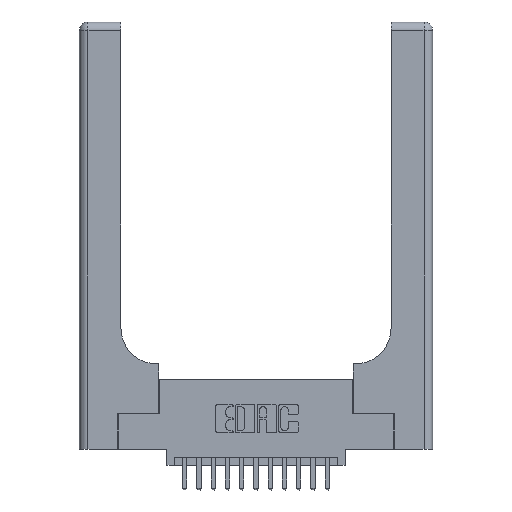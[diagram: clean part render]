
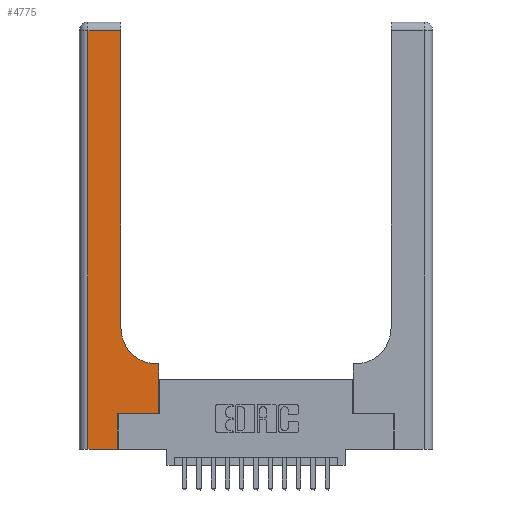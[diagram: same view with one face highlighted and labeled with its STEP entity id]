
A CAD part, top view. The second image highlights one B-rep face of the part: STEP entity #4775.
In plain terms, the highlighted planar face has unit normal (0, 0, 1).
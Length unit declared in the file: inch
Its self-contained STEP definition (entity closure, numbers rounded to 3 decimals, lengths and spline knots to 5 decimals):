
#497 = EDGE_CURVE ( 'NONE', #1761, #15109, #11783, .T. ) ;
#659 = DIRECTION ( 'NONE',  ( -1., 0., 0. ) ) ;
#733 = LINE ( 'NONE', #9240, #1203 ) ;
#1203 = VECTOR ( 'NONE', #659, 39.37008 ) ;
#1318 = DIRECTION ( 'NONE',  ( 0., 1., 0. ) ) ;
#1379 = CARTESIAN_POINT ( 'NONE',  ( 0., 2.94, 0.37 ) ) ;
#1761 = VERTEX_POINT ( 'NONE', #6984 ) ;
#1827 = LINE ( 'NONE', #14143, #13126 ) ;
#2099 = VERTEX_POINT ( 'NONE', #3879 ) ;
#2332 = DIRECTION ( 'NONE',  ( 0., 1., 0. ) ) ;
#2376 = VECTOR ( 'NONE', #1318, 39.37008 ) ;
#2440 = LINE ( 'NONE', #10809, #13709 ) ;
#2558 = VECTOR ( 'NONE', #11317, 39.37008 ) ;
#2577 = CIRCLE ( 'NONE', #3922, 0.25 ) ;
#2623 = PLANE ( 'NONE',  #12134 ) ;
#3007 = LINE ( 'NONE', #1379, #2558 ) ;
#3859 = VECTOR ( 'NONE', #8879, 39.37008 ) ;
#3879 = CARTESIAN_POINT ( 'NONE',  ( 0.5585, 0.6, 0.37 ) ) ;
#3919 = DIRECTION ( 'NONE',  ( 1., 0., 0. ) ) ;
#3922 = AXIS2_PLACEMENT_3D ( 'NONE', #13726, #5308, #15121 ) ;
#3931 = CARTESIAN_POINT ( 'NONE',  ( 0., 0., 0.37 ) ) ;
#3990 = DIRECTION ( 'NONE',  ( 1., 0., 0. ) ) ;
#4253 = DIRECTION ( 'NONE',  ( 0., -1., 0. ) ) ;
#4258 = CARTESIAN_POINT ( 'NONE',  ( 0.5585, 0.25, 0.37 ) ) ;
#4658 = VERTEX_POINT ( 'NONE', #6550 ) ;
#4775 = ADVANCED_FACE ( 'NONE', ( #17881 ), #2623, .F. ) ;
#5308 = DIRECTION ( 'NONE',  ( 0., 0., -1. ) ) ;
#5500 = CARTESIAN_POINT ( 'NONE',  ( 0.269, 0.25, 0.37 ) ) ;
#5503 = DIRECTION ( 'NONE',  ( 0., 0., -1. ) ) ;
#6205 = VECTOR ( 'NONE', #3990, 39.37008 ) ;
#6450 = CARTESIAN_POINT ( 'NONE',  ( 0.2915, 2.94, 0.37 ) ) ;
#6550 = CARTESIAN_POINT ( 'NONE',  ( 0.5585, 0.25, 0.37 ) ) ;
#6673 = EDGE_CURVE ( 'NONE', #6721, #1761, #17290, .T. ) ;
#6721 = VERTEX_POINT ( 'NONE', #6948 ) ;
#6804 = EDGE_LOOP ( 'NONE', ( #8723, #9300, #10432, #13533, #15608, #15686, #16881, #18004, #18183 ) ) ;
#6948 = CARTESIAN_POINT ( 'NONE',  ( 0.06, 0., 0.37 ) ) ;
#6984 = CARTESIAN_POINT ( 'NONE',  ( 0.269, 0., 0.37 ) ) ;
#7902 = EDGE_CURVE ( 'NONE', #16306, #13598, #2577, .T. ) ;
#8066 = CARTESIAN_POINT ( 'NONE',  ( 0.269, 0.25, 0.37 ) ) ;
#8712 = CARTESIAN_POINT ( 'NONE',  ( 0.269, 0., 0.37 ) ) ;
#8723 = ORIENTED_EDGE ( 'NONE', *, *, #12403, .T. ) ;
#8879 = DIRECTION ( 'NONE',  ( 0., 1., 0. ) ) ;
#9089 = EDGE_CURVE ( 'NONE', #12376, #11332, #3007, .T. ) ;
#9240 = CARTESIAN_POINT ( 'NONE',  ( 0.2915, 0.6, 0.37 ) ) ;
#9300 = ORIENTED_EDGE ( 'NONE', *, *, #9089, .T. ) ;
#9373 = CARTESIAN_POINT ( 'NONE',  ( 0.06, 2.94, 0.37 ) ) ;
#9928 = VECTOR ( 'NONE', #3919, 39.37008 ) ;
#10432 = ORIENTED_EDGE ( 'NONE', *, *, #16872, .T. ) ;
#10809 = CARTESIAN_POINT ( 'NONE',  ( 0.2915, 3., 0.37 ) ) ;
#11226 = CARTESIAN_POINT ( 'NONE',  ( 0.5415, 0.6, 0.37 ) ) ;
#11317 = DIRECTION ( 'NONE',  ( -1., 0., 0. ) ) ;
#11332 = VERTEX_POINT ( 'NONE', #9373 ) ;
#11783 = LINE ( 'NONE', #8712, #3859 ) ;
#12134 = AXIS2_PLACEMENT_3D ( 'NONE', #13912, #5503, #15293 ) ;
#12376 = VERTEX_POINT ( 'NONE', #6450 ) ;
#12403 = EDGE_CURVE ( 'NONE', #13598, #12376, #2440, .T. ) ;
#13126 = VECTOR ( 'NONE', #4253, 39.37008 ) ;
#13533 = ORIENTED_EDGE ( 'NONE', *, *, #6673, .T. ) ;
#13598 = VERTEX_POINT ( 'NONE', #16106 ) ;
#13709 = VECTOR ( 'NONE', #2332, 39.37008 ) ;
#13726 = CARTESIAN_POINT ( 'NONE',  ( 0.5415, 0.85, 0.37 ) ) ;
#13851 = EDGE_CURVE ( 'NONE', #15109, #4658, #17283, .T. ) ;
#13912 = CARTESIAN_POINT ( 'NONE',  ( 0., 3., 0.37 ) ) ;
#14143 = CARTESIAN_POINT ( 'NONE',  ( 0.06, 3., 0.37 ) ) ;
#15109 = VERTEX_POINT ( 'NONE', #5500 ) ;
#15121 = DIRECTION ( 'NONE',  ( 1., 0., 0. ) ) ;
#15155 = EDGE_CURVE ( 'NONE', #4658, #2099, #16009, .T. ) ;
#15293 = DIRECTION ( 'NONE',  ( -1., 0., 0. ) ) ;
#15414 = EDGE_CURVE ( 'NONE', #2099, #16306, #733, .T. ) ;
#15608 = ORIENTED_EDGE ( 'NONE', *, *, #497, .T. ) ;
#15686 = ORIENTED_EDGE ( 'NONE', *, *, #13851, .T. ) ;
#16009 = LINE ( 'NONE', #4258, #2376 ) ;
#16106 = CARTESIAN_POINT ( 'NONE',  ( 0.2915, 0.85, 0.37 ) ) ;
#16306 = VERTEX_POINT ( 'NONE', #11226 ) ;
#16872 = EDGE_CURVE ( 'NONE', #11332, #6721, #1827, .T. ) ;
#16881 = ORIENTED_EDGE ( 'NONE', *, *, #15155, .T. ) ;
#17283 = LINE ( 'NONE', #8066, #9928 ) ;
#17290 = LINE ( 'NONE', #3931, #6205 ) ;
#17881 = FACE_OUTER_BOUND ( 'NONE', #6804, .T. ) ;
#18004 = ORIENTED_EDGE ( 'NONE', *, *, #15414, .T. ) ;
#18183 = ORIENTED_EDGE ( 'NONE', *, *, #7902, .T. ) ;
